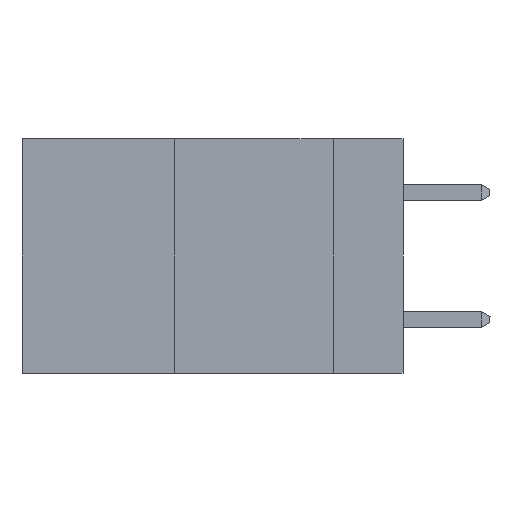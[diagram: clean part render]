
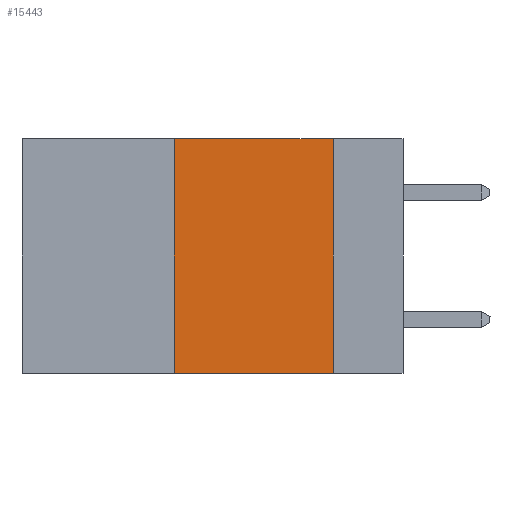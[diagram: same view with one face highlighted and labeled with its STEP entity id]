
A CAD part, left-side view. The second image highlights one B-rep face of the part: STEP entity #15443.
In plain terms, the highlighted planar face has unit normal (-1, 0, 0).
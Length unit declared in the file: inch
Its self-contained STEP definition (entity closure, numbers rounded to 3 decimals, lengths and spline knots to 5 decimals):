
#504 = CARTESIAN_POINT ( 'NONE',  ( 0., 0.11, 0. ) ) ;
#541 = ORIENTED_EDGE ( 'NONE', *, *, #23109, .F. ) ;
#566 = VERTEX_POINT ( 'NONE', #7353 ) ;
#581 = VECTOR ( 'NONE', #14760, 39.37008 ) ;
#596 = DIRECTION ( 'NONE',  ( 0., 0., 1. ) ) ;
#1116 = CARTESIAN_POINT ( 'NONE',  ( 0., 0.11, 0. ) ) ;
#1223 = CARTESIAN_POINT ( 'NONE',  ( 0., 0.36, -0.37 ) ) ;
#3349 = AXIS2_PLACEMENT_3D ( 'NONE', #7393, #3965, #20254 ) ;
#3965 = DIRECTION ( 'NONE',  ( 1., 0., 0. ) ) ;
#4332 = ORIENTED_EDGE ( 'NONE', *, *, #10044, .F. ) ;
#4461 = CARTESIAN_POINT ( 'NONE',  ( 0., 0.36, 0. ) ) ;
#4939 = VECTOR ( 'NONE', #20660, 39.37008 ) ;
#5455 = CARTESIAN_POINT ( 'NONE',  ( 0., 0.6, 0. ) ) ;
#5766 = LINE ( 'NONE', #5455, #581 ) ;
#5936 = EDGE_CURVE ( 'NONE', #14970, #18666, #5766, .T. ) ;
#6012 = CARTESIAN_POINT ( 'NONE',  ( 0., 0.6, -0.37 ) ) ;
#6988 = VECTOR ( 'NONE', #596, 39.37008 ) ;
#7353 = CARTESIAN_POINT ( 'NONE',  ( 0., 0.11, -0.37 ) ) ;
#7393 = CARTESIAN_POINT ( 'NONE',  ( 0., 0.6, 0. ) ) ;
#8331 = VECTOR ( 'NONE', #17706, 39.37008 ) ;
#10044 = EDGE_CURVE ( 'NONE', #18666, #566, #13243, .T. ) ;
#10872 = VERTEX_POINT ( 'NONE', #1223 ) ;
#11025 = LINE ( 'NONE', #6012, #4939 ) ;
#11349 = EDGE_CURVE ( 'NONE', #10872, #566, #11025, .T. ) ;
#12197 = LINE ( 'NONE', #4461, #6988 ) ;
#13243 = LINE ( 'NONE', #1116, #8331 ) ;
#14760 = DIRECTION ( 'NONE',  ( 0., -1., 0. ) ) ;
#14962 = FACE_OUTER_BOUND ( 'NONE', #16223, .T. ) ;
#14970 = VERTEX_POINT ( 'NONE', #19935 ) ;
#15443 = ADVANCED_FACE ( 'NONE', ( #14962 ), #18623, .F. ) ;
#16223 = EDGE_LOOP ( 'NONE', ( #4332, #17585, #541, #21998 ) ) ;
#17585 = ORIENTED_EDGE ( 'NONE', *, *, #5936, .F. ) ;
#17706 = DIRECTION ( 'NONE',  ( 0., 0., -1. ) ) ;
#18623 = PLANE ( 'NONE',  #3349 ) ;
#18666 = VERTEX_POINT ( 'NONE', #504 ) ;
#19935 = CARTESIAN_POINT ( 'NONE',  ( 0., 0.36, 0. ) ) ;
#20254 = DIRECTION ( 'NONE',  ( 0., 0., -1. ) ) ;
#20660 = DIRECTION ( 'NONE',  ( 0., -1., 0. ) ) ;
#21998 = ORIENTED_EDGE ( 'NONE', *, *, #11349, .T. ) ;
#23109 = EDGE_CURVE ( 'NONE', #10872, #14970, #12197, .T. ) ;
